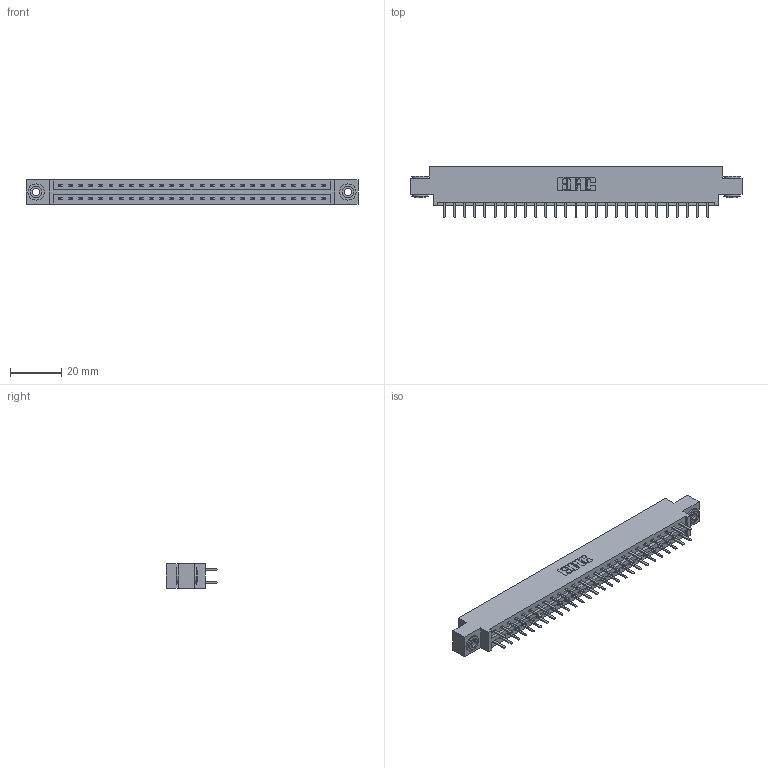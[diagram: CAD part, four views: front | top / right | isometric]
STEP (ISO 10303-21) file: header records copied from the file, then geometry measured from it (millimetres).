
FILE_DESCRIPTION (( 'STEP AP203' ), '1' );
FILE_NAME ('387-054-520-803.STEP', '2018-09-20T21:49:03', ( '' ), ( '' ), 'SwSTEP 2.0', 'SolidWorks 2016', '' );
FILE_SCHEMA (( 'CONFIG_CONTROL_DESIGN' ));
Length unit declared in the file: inch
Products named in the file (4): 337 Part_0.170 Offset - 0.156 Dia-TH; 345-292-001_345-293-120; 345-250-002_345-250-002-102; 387-054-520-803
Assembly tree (57 placements, depth 2):
  387-054-520-803
    337 Part_0.170 Offset - 0.156 Dia-TH
    345-292-001_345-293-120  x54
    345-250-002_345-250-002-102  x2
Bounding box: 130 x 20.02 x 9.4 mm (x, y, z)
Volume: 13378.6 mm3; surface area: 15243.4 mm2
Topology: 57 solids, 57 shells, 3288 faces, 9525 edges, 6202 vertices
Faces by surface type: plane 2244, cylinder 1036, cone 8
Entity records: 23770 total; most frequent: CARTESIAN_POINT 4005, ORIENTED_EDGE 3922, DIRECTION 3455, EDGE_CURVE 1961, VECTOR 1805, LINE 1805, VERTEX_POINT 1302, AXIS2_PLACEMENT_3D 825
